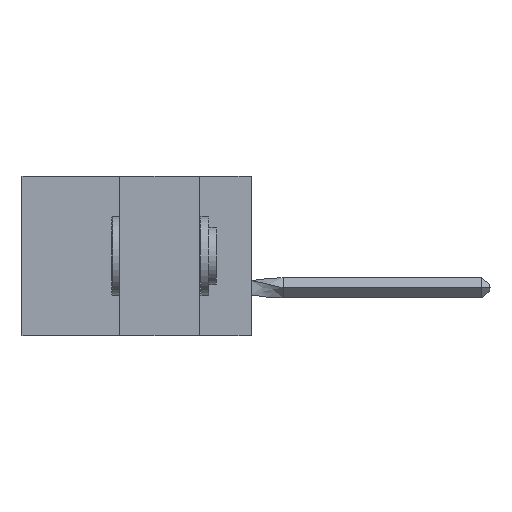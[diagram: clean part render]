
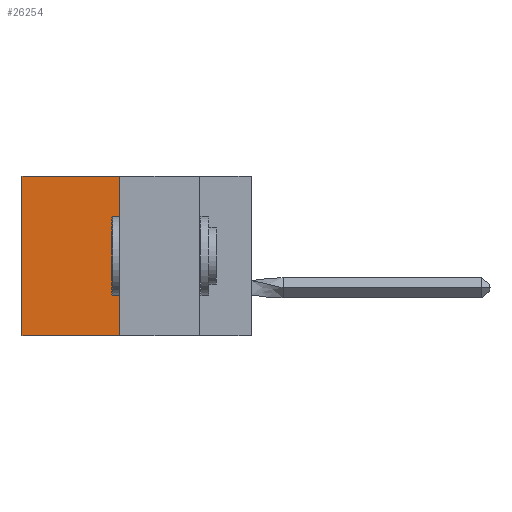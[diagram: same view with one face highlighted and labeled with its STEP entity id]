
A CAD part, left-side view. The second image highlights one B-rep face of the part: STEP entity #26254.
In plain terms, the highlighted planar face has unit normal (-1, 0, 0).
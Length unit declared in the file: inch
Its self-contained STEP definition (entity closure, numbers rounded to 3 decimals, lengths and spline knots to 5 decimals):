
#294 = EDGE_LOOP ( 'NONE', ( #21079, #6095, #41553, #9917 ) ) ;
#4997 = CARTESIAN_POINT ( 'NONE',  ( 0.305, 0.413, -0.5 ) ) ;
#5720 = CARTESIAN_POINT ( 'NONE',  ( 0.305, 0.72, 0. ) ) ;
#6095 = ORIENTED_EDGE ( 'NONE', *, *, #38842, .F. ) ;
#6354 = VECTOR ( 'NONE', #10279, 39.37008 ) ;
#6765 = VECTOR ( 'NONE', #31375, 39.37008 ) ;
#6897 = DIRECTION ( 'NONE',  ( 0., 1., 0. ) ) ;
#7333 = CARTESIAN_POINT ( 'NONE',  ( 0.305, 0.413, -0.5 ) ) ;
#8102 = PLANE ( 'NONE',  #23874 ) ;
#8183 = CARTESIAN_POINT ( 'NONE',  ( 0.305, 0.72, -0.5 ) ) ;
#9917 = ORIENTED_EDGE ( 'NONE', *, *, #32727, .T. ) ;
#10279 = DIRECTION ( 'NONE',  ( 0., 1., 0. ) ) ;
#12505 = LINE ( 'NONE', #35365, #23740 ) ;
#12858 = FACE_OUTER_BOUND ( 'NONE', #294, .T. ) ;
#13766 = EDGE_CURVE ( 'NONE', #29869, #39131, #24206, .T. ) ;
#13902 = CARTESIAN_POINT ( 'NONE',  ( 0.305, 0.413, 0. ) ) ;
#15106 = CARTESIAN_POINT ( 'NONE',  ( 0.305, 0.72, -0.5 ) ) ;
#15944 = VECTOR ( 'NONE', #6897, 39.37008 ) ;
#18023 = LINE ( 'NONE', #7333, #15944 ) ;
#20737 = CARTESIAN_POINT ( 'NONE',  ( 0.305, 0.413, -0.5 ) ) ;
#21079 = ORIENTED_EDGE ( 'NONE', *, *, #13766, .T. ) ;
#23740 = VECTOR ( 'NONE', #38663, 39.37008 ) ;
#23874 = AXIS2_PLACEMENT_3D ( 'NONE', #20737, #27251, #30849 ) ;
#24206 = LINE ( 'NONE', #15106, #6765 ) ;
#26254 = ADVANCED_FACE ( 'NONE', ( #12858 ), #8102, .F. ) ;
#27251 = DIRECTION ( 'NONE',  ( 1., 0., 0. ) ) ;
#29869 = VERTEX_POINT ( 'NONE', #5720 ) ;
#30849 = DIRECTION ( 'NONE',  ( 0., 0., -1. ) ) ;
#31375 = DIRECTION ( 'NONE',  ( 0., 0., -1. ) ) ;
#32727 = EDGE_CURVE ( 'NONE', #37345, #29869, #33522, .T. ) ;
#33522 = LINE ( 'NONE', #13902, #6354 ) ;
#35365 = CARTESIAN_POINT ( 'NONE',  ( 0.305, 0.413, -0.5 ) ) ;
#36936 = EDGE_CURVE ( 'NONE', #37345, #38005, #12505, .T. ) ;
#37345 = VERTEX_POINT ( 'NONE', #41464 ) ;
#38005 = VERTEX_POINT ( 'NONE', #4997 ) ;
#38663 = DIRECTION ( 'NONE',  ( 0., 0., -1. ) ) ;
#38842 = EDGE_CURVE ( 'NONE', #38005, #39131, #18023, .T. ) ;
#39131 = VERTEX_POINT ( 'NONE', #8183 ) ;
#41464 = CARTESIAN_POINT ( 'NONE',  ( 0.305, 0.413, 0. ) ) ;
#41553 = ORIENTED_EDGE ( 'NONE', *, *, #36936, .F. ) ;
